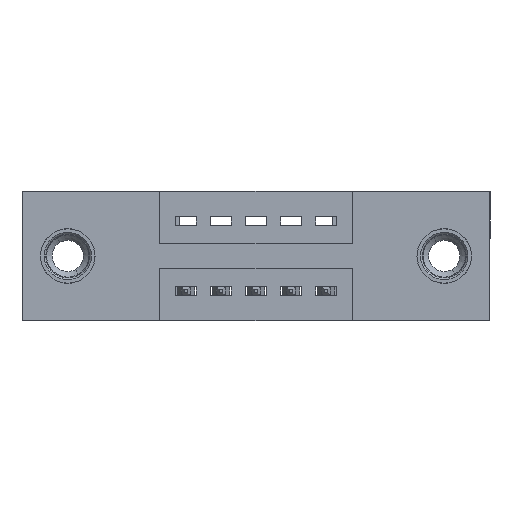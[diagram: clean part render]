
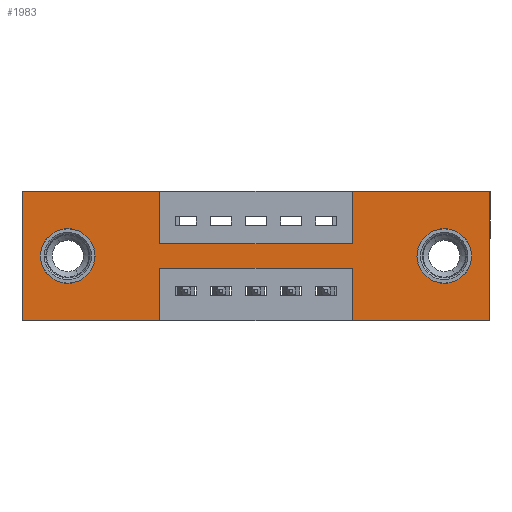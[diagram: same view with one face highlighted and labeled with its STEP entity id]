
A CAD part, front view. The second image highlights one B-rep face of the part: STEP entity #1983.
In plain terms, the highlighted planar face has unit normal (0, -1, 0).
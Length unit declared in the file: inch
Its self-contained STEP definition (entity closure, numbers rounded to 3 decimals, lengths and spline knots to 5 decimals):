
#58 = ORIENTED_EDGE ( 'NONE', *, *, #7912, .F. ) ;
#161 = FACE_BOUND ( 'NONE', #9138, .T. ) ;
#194 = CIRCLE ( 'NONE', #1525, 0.078 ) ;
#244 = CARTESIAN_POINT ( 'NONE',  ( 0.9425, 0., 0. ) ) ;
#306 = EDGE_CURVE ( 'NONE', #6115, #2612, #10373, .T. ) ;
#533 = VECTOR ( 'NONE', #6354, 39.37008 ) ;
#762 = CARTESIAN_POINT ( 'NONE',  ( 0.13, 0., -0.185 ) ) ;
#885 = ORIENTED_EDGE ( 'NONE', *, *, #10282, .T. ) ;
#942 = VECTOR ( 'NONE', #1651, 39.37008 ) ;
#997 = AXIS2_PLACEMENT_3D ( 'NONE', #7236, #7270, #8007 ) ;
#1069 = LINE ( 'NONE', #1530, #7524 ) ;
#1311 = VERTEX_POINT ( 'NONE', #9717 ) ;
#1313 = AXIS2_PLACEMENT_3D ( 'NONE', #7853, #5366, #9645 ) ;
#1525 = AXIS2_PLACEMENT_3D ( 'NONE', #10051, #6618, #1563 ) ;
#1530 = CARTESIAN_POINT ( 'NONE',  ( 0.9425, 0., -0.37 ) ) ;
#1563 = DIRECTION ( 'NONE',  ( 0., 0., -1. ) ) ;
#1624 = CARTESIAN_POINT ( 'NONE',  ( 0.3925, 0., -0.22 ) ) ;
#1651 = DIRECTION ( 'NONE',  ( 1., 0., 0. ) ) ;
#1842 = EDGE_CURVE ( 'NONE', #8131, #4272, #10852, .T. ) ;
#1904 = EDGE_LOOP ( 'NONE', ( #2016, #10318, #9550, #5003, #3237, #5804, #6101, #58, #8549, #6782, #9431, #7354 ) ) ;
#1983 = ADVANCED_FACE ( 'NONE', ( #161, #8468, #2155 ), #2873, .T. ) ;
#2016 = ORIENTED_EDGE ( 'NONE', *, *, #8065, .F. ) ;
#2155 = FACE_OUTER_BOUND ( 'NONE', #1904, .T. ) ;
#2207 = VERTEX_POINT ( 'NONE', #2628 ) ;
#2360 = VERTEX_POINT ( 'NONE', #7555 ) ;
#2398 = DIRECTION ( 'NONE',  ( 0., 0., 1. ) ) ;
#2436 = VECTOR ( 'NONE', #5469, 39.37008 ) ;
#2547 = CARTESIAN_POINT ( 'NONE',  ( 1.335, 0., -0.37 ) ) ;
#2591 = CARTESIAN_POINT ( 'NONE',  ( 0.9425, 0., 0. ) ) ;
#2602 = DIRECTION ( 'NONE',  ( -1., 0., 0. ) ) ;
#2612 = VERTEX_POINT ( 'NONE', #5072 ) ;
#2628 = CARTESIAN_POINT ( 'NONE',  ( 0.3925, 0., 0. ) ) ;
#2839 = CARTESIAN_POINT ( 'NONE',  ( 0., 0., -0.37 ) ) ;
#2873 = PLANE ( 'NONE',  #1313 ) ;
#3044 = ORIENTED_EDGE ( 'NONE', *, *, #5899, .T. ) ;
#3085 = VERTEX_POINT ( 'NONE', #9800 ) ;
#3176 = LINE ( 'NONE', #10062, #942 ) ;
#3237 = ORIENTED_EDGE ( 'NONE', *, *, #10725, .F. ) ;
#3346 = DIRECTION ( 'NONE',  ( 0., 0., -1. ) ) ;
#3443 = DIRECTION ( 'NONE',  ( 0., 0., 1. ) ) ;
#3653 = EDGE_CURVE ( 'NONE', #2207, #2360, #10097, .T. ) ;
#3928 = VECTOR ( 'NONE', #6016, 39.37008 ) ;
#4076 = CIRCLE ( 'NONE', #6249, 0.078 ) ;
#4100 = CARTESIAN_POINT ( 'NONE',  ( 0.9425, 0., -0.37 ) ) ;
#4191 = DIRECTION ( 'NONE',  ( -1., 0., 0. ) ) ;
#4231 = LINE ( 'NONE', #8685, #9813 ) ;
#4272 = VERTEX_POINT ( 'NONE', #1624 ) ;
#4560 = EDGE_CURVE ( 'NONE', #2612, #9164, #8782, .T. ) ;
#4856 = CARTESIAN_POINT ( 'NONE',  ( 0., 0., 0. ) ) ;
#4911 = ORIENTED_EDGE ( 'NONE', *, *, #6786, .T. ) ;
#5003 = ORIENTED_EDGE ( 'NONE', *, *, #5369, .F. ) ;
#5005 = CARTESIAN_POINT ( 'NONE',  ( 1.205, 0., -0.263 ) ) ;
#5072 = CARTESIAN_POINT ( 'NONE',  ( 0., 0., -0.37 ) ) ;
#5130 = CARTESIAN_POINT ( 'NONE',  ( 0.9425, 0., -0.22 ) ) ;
#5269 = LINE ( 'NONE', #10381, #3928 ) ;
#5317 = CARTESIAN_POINT ( 'NONE',  ( 0.3925, 0., 0. ) ) ;
#5348 = VERTEX_POINT ( 'NONE', #6104 ) ;
#5366 = DIRECTION ( 'NONE',  ( 0., -1., 0. ) ) ;
#5369 = EDGE_CURVE ( 'NONE', #8668, #7211, #10211, .T. ) ;
#5469 = DIRECTION ( 'NONE',  ( 0., 0., -1. ) ) ;
#5664 = EDGE_CURVE ( 'NONE', #7557, #10580, #9140, .T. ) ;
#5700 = VECTOR ( 'NONE', #7054, 39.37008 ) ;
#5706 = DIRECTION ( 'NONE',  ( 0., 1., 0. ) ) ;
#5733 = VECTOR ( 'NONE', #3443, 39.37008 ) ;
#5804 = ORIENTED_EDGE ( 'NONE', *, *, #6336, .F. ) ;
#5899 = EDGE_CURVE ( 'NONE', #8344, #1311, #10711, .T. ) ;
#5937 = CARTESIAN_POINT ( 'NONE',  ( 0.3925, 0., -0.22 ) ) ;
#6016 = DIRECTION ( 'NONE',  ( 1., 0., 0. ) ) ;
#6101 = ORIENTED_EDGE ( 'NONE', *, *, #5664, .F. ) ;
#6104 = CARTESIAN_POINT ( 'NONE',  ( 1.335, 0., 0. ) ) ;
#6115 = VERTEX_POINT ( 'NONE', #10059 ) ;
#6249 = AXIS2_PLACEMENT_3D ( 'NONE', #762, #7480, #10828 ) ;
#6336 = EDGE_CURVE ( 'NONE', #10580, #5348, #9129, .T. ) ;
#6354 = DIRECTION ( 'NONE',  ( 1., 0., 0. ) ) ;
#6425 = ORIENTED_EDGE ( 'NONE', *, *, #9315, .T. ) ;
#6510 = EDGE_CURVE ( 'NONE', #7211, #8131, #1069, .T. ) ;
#6618 = DIRECTION ( 'NONE',  ( 0., 1., 0. ) ) ;
#6782 = ORIENTED_EDGE ( 'NONE', *, *, #10538, .F. ) ;
#6786 = EDGE_CURVE ( 'NONE', #1311, #8344, #4076, .T. ) ;
#6946 = DIRECTION ( 'NONE',  ( -1., 0., 0. ) ) ;
#7054 = DIRECTION ( 'NONE',  ( 0., 0., 1. ) ) ;
#7211 = VERTEX_POINT ( 'NONE', #4100 ) ;
#7236 = CARTESIAN_POINT ( 'NONE',  ( 1.205, 0., -0.185 ) ) ;
#7270 = DIRECTION ( 'NONE',  ( 0., 1., 0. ) ) ;
#7354 = ORIENTED_EDGE ( 'NONE', *, *, #306, .F. ) ;
#7368 = DIRECTION ( 'NONE',  ( 0., 0., 1. ) ) ;
#7480 = DIRECTION ( 'NONE',  ( 0., 1., 0. ) ) ;
#7524 = VECTOR ( 'NONE', #2398, 39.37008 ) ;
#7543 = CARTESIAN_POINT ( 'NONE',  ( 0.13, 0., -0.263 ) ) ;
#7555 = CARTESIAN_POINT ( 'NONE',  ( 0.3925, 0., -0.15 ) ) ;
#7557 = VERTEX_POINT ( 'NONE', #10260 ) ;
#7853 = CARTESIAN_POINT ( 'NONE',  ( 0., 0., -0.37 ) ) ;
#7912 = EDGE_CURVE ( 'NONE', #2360, #7557, #5269, .T. ) ;
#7954 = VECTOR ( 'NONE', #6946, 39.37008 ) ;
#8007 = DIRECTION ( 'NONE',  ( 0., 0., -1. ) ) ;
#8065 = EDGE_CURVE ( 'NONE', #4272, #6115, #10534, .T. ) ;
#8078 = CARTESIAN_POINT ( 'NONE',  ( 0., 0., 0. ) ) ;
#8131 = VERTEX_POINT ( 'NONE', #5130 ) ;
#8344 = VERTEX_POINT ( 'NONE', #7543 ) ;
#8468 = FACE_BOUND ( 'NONE', #10417, .T. ) ;
#8549 = ORIENTED_EDGE ( 'NONE', *, *, #3653, .F. ) ;
#8566 = CARTESIAN_POINT ( 'NONE',  ( 0., 0., 0. ) ) ;
#8611 = DIRECTION ( 'NONE',  ( 0., 0., -1. ) ) ;
#8668 = VERTEX_POINT ( 'NONE', #2547 ) ;
#8685 = CARTESIAN_POINT ( 'NONE',  ( 1.335, 0., 0. ) ) ;
#8782 = LINE ( 'NONE', #8566, #5733 ) ;
#8919 = VECTOR ( 'NONE', #4191, 39.37008 ) ;
#9129 = LINE ( 'NONE', #8078, #533 ) ;
#9138 = EDGE_LOOP ( 'NONE', ( #6425, #885 ) ) ;
#9140 = LINE ( 'NONE', #244, #5700 ) ;
#9164 = VERTEX_POINT ( 'NONE', #4856 ) ;
#9181 = CARTESIAN_POINT ( 'NONE',  ( 0.13, 0., -0.185 ) ) ;
#9315 = EDGE_CURVE ( 'NONE', #3085, #10560, #194, .T. ) ;
#9334 = CARTESIAN_POINT ( 'NONE',  ( 0., 0., -0.37 ) ) ;
#9349 = VECTOR ( 'NONE', #3346, 39.37008 ) ;
#9431 = ORIENTED_EDGE ( 'NONE', *, *, #4560, .F. ) ;
#9510 = AXIS2_PLACEMENT_3D ( 'NONE', #9181, #5706, #7368 ) ;
#9550 = ORIENTED_EDGE ( 'NONE', *, *, #6510, .F. ) ;
#9645 = DIRECTION ( 'NONE',  ( 0., 0., -1. ) ) ;
#9717 = CARTESIAN_POINT ( 'NONE',  ( 0.13, 0., -0.107 ) ) ;
#9800 = CARTESIAN_POINT ( 'NONE',  ( 1.205, 0., -0.107 ) ) ;
#9813 = VECTOR ( 'NONE', #8611, 39.37008 ) ;
#10051 = CARTESIAN_POINT ( 'NONE',  ( 1.205, 0., -0.185 ) ) ;
#10059 = CARTESIAN_POINT ( 'NONE',  ( 0.3925, 0., -0.37 ) ) ;
#10062 = CARTESIAN_POINT ( 'NONE',  ( 0., 0., 0. ) ) ;
#10097 = LINE ( 'NONE', #5317, #2436 ) ;
#10211 = LINE ( 'NONE', #2839, #7954 ) ;
#10260 = CARTESIAN_POINT ( 'NONE',  ( 0.9425, 0., -0.15 ) ) ;
#10282 = EDGE_CURVE ( 'NONE', #10560, #3085, #10472, .T. ) ;
#10318 = ORIENTED_EDGE ( 'NONE', *, *, #1842, .F. ) ;
#10356 = VECTOR ( 'NONE', #2602, 39.37008 ) ;
#10373 = LINE ( 'NONE', #9334, #8919 ) ;
#10381 = CARTESIAN_POINT ( 'NONE',  ( 0.3925, 0., -0.15 ) ) ;
#10417 = EDGE_LOOP ( 'NONE', ( #4911, #3044 ) ) ;
#10472 = CIRCLE ( 'NONE', #997, 0.078 ) ;
#10534 = LINE ( 'NONE', #10907, #9349 ) ;
#10538 = EDGE_CURVE ( 'NONE', #9164, #2207, #3176, .T. ) ;
#10560 = VERTEX_POINT ( 'NONE', #5005 ) ;
#10580 = VERTEX_POINT ( 'NONE', #2591 ) ;
#10711 = CIRCLE ( 'NONE', #9510, 0.078 ) ;
#10725 = EDGE_CURVE ( 'NONE', #5348, #8668, #4231, .T. ) ;
#10828 = DIRECTION ( 'NONE',  ( 0., 0., 1. ) ) ;
#10852 = LINE ( 'NONE', #5937, #10356 ) ;
#10907 = CARTESIAN_POINT ( 'NONE',  ( 0.3925, 0., -0.37 ) ) ;
